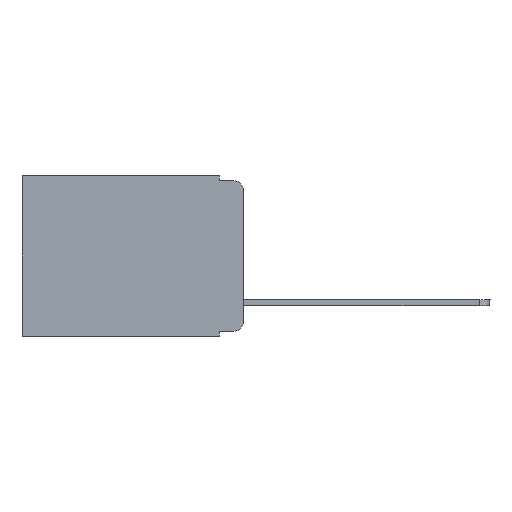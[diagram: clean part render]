
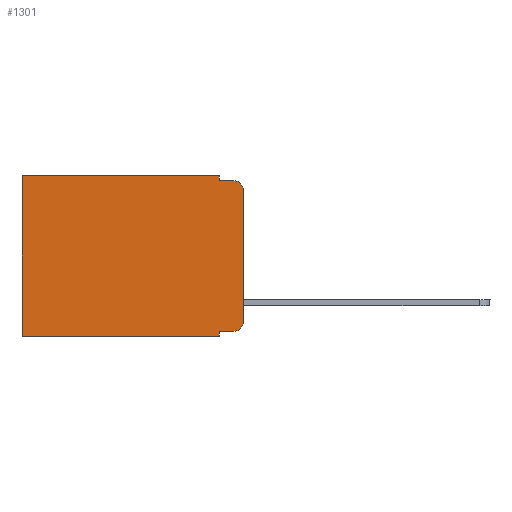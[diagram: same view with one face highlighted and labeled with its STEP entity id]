
A CAD part, left-side view. The second image highlights one B-rep face of the part: STEP entity #1301.
In plain terms, the highlighted planar face has unit normal (-1, 0, 0).
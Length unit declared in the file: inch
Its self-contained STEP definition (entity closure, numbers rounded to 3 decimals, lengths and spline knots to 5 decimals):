
#68 = LINE ( 'NONE', #13891, #14332 ) ;
#174 = CARTESIAN_POINT ( 'NONE',  ( 0.298, 0.473, 0. ) ) ;
#201 = DIRECTION ( 'NONE',  ( -1., 0., 0. ) ) ;
#261 = CARTESIAN_POINT ( 'NONE',  ( 0.298, 0.051, -0.343 ) ) ;
#516 = ORIENTED_EDGE ( 'NONE', *, *, #11133, .F. ) ;
#819 = CARTESIAN_POINT ( 'NONE',  ( 0.298, 0.473, 0. ) ) ;
#1017 = AXIS2_PLACEMENT_3D ( 'NONE', #9568, #6646, #3993 ) ;
#1073 = CARTESIAN_POINT ( 'NONE',  ( 0.298, 0., 0. ) ) ;
#1230 = EDGE_CURVE ( 'NONE', #4456, #15713, #2257, .T. ) ;
#1301 = ADVANCED_FACE ( 'NONE', ( #13774 ), #2792, .F. ) ;
#1303 = CARTESIAN_POINT ( 'NONE',  ( 0.298, 0.051, -0.01 ) ) ;
#1440 = DIRECTION ( 'NONE',  ( 0., -1., 0. ) ) ;
#1486 = VECTOR ( 'NONE', #17294, 39.37008 ) ;
#1515 = ORIENTED_EDGE ( 'NONE', *, *, #4726, .F. ) ;
#1602 = VECTOR ( 'NONE', #8424, 39.37008 ) ;
#2155 = AXIS2_PLACEMENT_3D ( 'NONE', #2945, #201, #8348 ) ;
#2257 = LINE ( 'NONE', #1073, #8579 ) ;
#2322 = ORIENTED_EDGE ( 'NONE', *, *, #15908, .T. ) ;
#2338 = VERTEX_POINT ( 'NONE', #7885 ) ;
#2474 = VECTOR ( 'NONE', #1440, 39.37008 ) ;
#2490 = EDGE_CURVE ( 'NONE', #4456, #2338, #15208, .T. ) ;
#2654 = DIRECTION ( 'NONE',  ( 0., 0., -1. ) ) ;
#2742 = VERTEX_POINT ( 'NONE', #6655 ) ;
#2792 = PLANE ( 'NONE',  #1017 ) ;
#2847 = CARTESIAN_POINT ( 'NONE',  ( 0.298, 0.051, 0. ) ) ;
#2945 = CARTESIAN_POINT ( 'NONE',  ( 0.298, 0.02, -0.313 ) ) ;
#3379 = LINE ( 'NONE', #13167, #1486 ) ;
#3993 = DIRECTION ( 'NONE',  ( 0., 0., -1. ) ) ;
#4456 = VERTEX_POINT ( 'NONE', #5809 ) ;
#4726 = EDGE_CURVE ( 'NONE', #2338, #10732, #11002, .T. ) ;
#5476 = EDGE_CURVE ( 'NONE', #2742, #15972, #9324, .T. ) ;
#5809 = CARTESIAN_POINT ( 'NONE',  ( 0.298, 0.051, 0. ) ) ;
#5812 = DIRECTION ( 'NONE',  ( 0., 0., -1. ) ) ;
#5895 = CARTESIAN_POINT ( 'NONE',  ( 0.298, 0.02, -0.03 ) ) ;
#5902 = CARTESIAN_POINT ( 'NONE',  ( 0.298, 0.473, -0.343 ) ) ;
#6402 = ORIENTED_EDGE ( 'NONE', *, *, #15088, .T. ) ;
#6646 = DIRECTION ( 'NONE',  ( 1., 0., 0. ) ) ;
#6655 = CARTESIAN_POINT ( 'NONE',  ( 0.298, 0., -0.03 ) ) ;
#6881 = VECTOR ( 'NONE', #7659, 39.37008 ) ;
#6955 = CARTESIAN_POINT ( 'NONE',  ( 0.298, 0.02, -0.01 ) ) ;
#7567 = VERTEX_POINT ( 'NONE', #5902 ) ;
#7659 = DIRECTION ( 'NONE',  ( 0., 0., -1. ) ) ;
#7683 = VERTEX_POINT ( 'NONE', #13380 ) ;
#7885 = CARTESIAN_POINT ( 'NONE',  ( 0.298, 0.051, -0.01 ) ) ;
#8348 = DIRECTION ( 'NONE',  ( 0., 0., -1. ) ) ;
#8424 = DIRECTION ( 'NONE',  ( 0., 0., -1. ) ) ;
#8579 = VECTOR ( 'NONE', #13414, 39.37008 ) ;
#9142 = ORIENTED_EDGE ( 'NONE', *, *, #5476, .F. ) ;
#9324 = LINE ( 'NONE', #14536, #6881 ) ;
#9532 = VECTOR ( 'NONE', #9878, 39.37008 ) ;
#9568 = CARTESIAN_POINT ( 'NONE',  ( 0.298, 0., 0. ) ) ;
#9678 = DIRECTION ( 'NONE',  ( 0., 0., -1. ) ) ;
#9685 = LINE ( 'NONE', #174, #9691 ) ;
#9691 = VECTOR ( 'NONE', #2654, 39.37008 ) ;
#9731 = DIRECTION ( 'NONE',  ( -1., 0., 0. ) ) ;
#9878 = DIRECTION ( 'NONE',  ( 0., -1., 0. ) ) ;
#10250 = VERTEX_POINT ( 'NONE', #10640 ) ;
#10640 = CARTESIAN_POINT ( 'NONE',  ( 0.298, 0.02, -0.333 ) ) ;
#10648 = ORIENTED_EDGE ( 'NONE', *, *, #2490, .F. ) ;
#10732 = VERTEX_POINT ( 'NONE', #6955 ) ;
#11002 = LINE ( 'NONE', #1303, #9532 ) ;
#11133 = EDGE_CURVE ( 'NONE', #7683, #13778, #68, .T. ) ;
#11490 = CIRCLE ( 'NONE', #2155, 0.02 ) ;
#11926 = CARTESIAN_POINT ( 'NONE',  ( 0.298, 0., -0.313 ) ) ;
#12197 = EDGE_CURVE ( 'NONE', #13778, #7567, #3379, .T. ) ;
#12516 = CARTESIAN_POINT ( 'NONE',  ( 0.298, 0.051, -0.333 ) ) ;
#13167 = CARTESIAN_POINT ( 'NONE',  ( 0.298, 0., -0.343 ) ) ;
#13380 = CARTESIAN_POINT ( 'NONE',  ( 0.298, 0.051, -0.333 ) ) ;
#13414 = DIRECTION ( 'NONE',  ( 0., 1., 0. ) ) ;
#13696 = EDGE_CURVE ( 'NONE', #15713, #7567, #9685, .T. ) ;
#13774 = FACE_OUTER_BOUND ( 'NONE', #17483, .T. ) ;
#13778 = VERTEX_POINT ( 'NONE', #261 ) ;
#13891 = CARTESIAN_POINT ( 'NONE',  ( 0.298, 0.051, 0. ) ) ;
#13977 = LINE ( 'NONE', #12516, #2474 ) ;
#14332 = VECTOR ( 'NONE', #9678, 39.37008 ) ;
#14400 = AXIS2_PLACEMENT_3D ( 'NONE', #5895, #9731, #5812 ) ;
#14536 = CARTESIAN_POINT ( 'NONE',  ( 0.298, 0., 0. ) ) ;
#14639 = EDGE_CURVE ( 'NONE', #2742, #10732, #16458, .T. ) ;
#14644 = ORIENTED_EDGE ( 'NONE', *, *, #12197, .F. ) ;
#15088 = EDGE_CURVE ( 'NONE', #10250, #15972, #11490, .T. ) ;
#15208 = LINE ( 'NONE', #2847, #1602 ) ;
#15713 = VERTEX_POINT ( 'NONE', #819 ) ;
#15908 = EDGE_CURVE ( 'NONE', #7683, #10250, #13977, .T. ) ;
#15972 = VERTEX_POINT ( 'NONE', #11926 ) ;
#16437 = ORIENTED_EDGE ( 'NONE', *, *, #13696, .T. ) ;
#16458 = CIRCLE ( 'NONE', #14400, 0.02 ) ;
#16734 = ORIENTED_EDGE ( 'NONE', *, *, #14639, .T. ) ;
#17191 = ORIENTED_EDGE ( 'NONE', *, *, #1230, .T. ) ;
#17294 = DIRECTION ( 'NONE',  ( 0., 1., 0. ) ) ;
#17483 = EDGE_LOOP ( 'NONE', ( #9142, #16734, #1515, #10648, #17191, #16437, #14644, #516, #2322, #6402 ) ) ;
